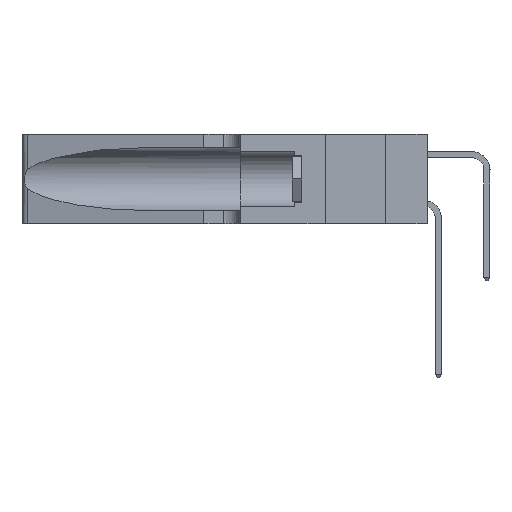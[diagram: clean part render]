
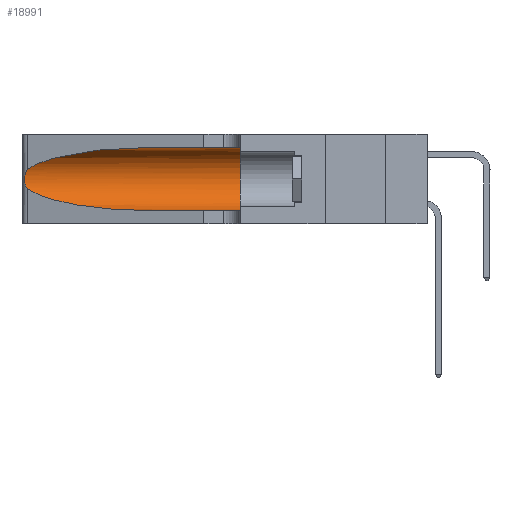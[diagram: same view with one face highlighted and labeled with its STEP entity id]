
A CAD part, left-side view. The second image highlights one B-rep face of the part: STEP entity #18991.
In plain terms, the highlighted cylindrical face has radius 3.308 mm (diameter 6.617 mm), a partial arc.
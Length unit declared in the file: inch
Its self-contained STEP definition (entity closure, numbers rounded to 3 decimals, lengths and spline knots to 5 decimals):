
#11 = EDGE_CURVE ( 'NONE', #18755, #27238, #30736, .T. ) ;
#46 = DIRECTION ( 'NONE',  ( 0., 1., 0. ) ) ;
#856 = CARTESIAN_POINT ( 'NONE',  ( 0.1305, 0.35, 0.05475 ) ) ;
#1956 = CARTESIAN_POINT ( 'NONE',  ( 0.25787, 1.23484, 0.2124 ) ) ;
#2118 = ORIENTED_EDGE ( 'NONE', *, *, #9634, .F. ) ;
#4438 = LINE ( 'NONE', #8211, #25251 ) ;
#4688 = CARTESIAN_POINT ( 'NONE',  ( 0.26018, 1.23835, 0.19895 ) ) ;
#5260 = ORIENTED_EDGE ( 'NONE', *, *, #29958, .T. ) ;
#6292 = CARTESIAN_POINT ( 'NONE',  ( 0.1305, 1.61858, 0.31525 ) ) ;
#6932 = EDGE_CURVE ( 'NONE', #11628, #14616, #9971, .T. ) ;
#7225 = DIRECTION ( 'NONE',  ( 0., 0., -1. ) ) ;
#7465 = CARTESIAN_POINT ( 'NONE',  ( 0.26075, 1.23896, 0.178 ) ) ;
#8211 = CARTESIAN_POINT ( 'NONE',  ( 0.1305, 1.61858, 0.05475 ) ) ;
#8562 = CARTESIAN_POINT ( 'NONE',  ( 0.1305, 0.35, 0.31525 ) ) ;
#8571 = VERTEX_POINT ( 'NONE', #21417 ) ;
#8962 = CARTESIAN_POINT ( 'NONE',  ( 0.1305, 0.35, 0.185 ) ) ;
#9035 = FACE_OUTER_BOUND ( 'NONE', #20756, .T. ) ;
#9094 = CARTESIAN_POINT ( 'NONE',  ( 0.18966, 0.96281, 0.31525 ) ) ;
#9478 = EDGE_CURVE ( 'NONE', #8571, #34686, #26212, .T. ) ;
#9634 = EDGE_CURVE ( 'NONE', #11628, #18755, #11579, .T. ) ;
#9971 =( BOUNDED_CURVE ( )  B_SPLINE_CURVE ( 3, ( #27988, #9094, #11837, #30648 ),
 .UNSPECIFIED., .F., .T. ) 
 B_SPLINE_CURVE_WITH_KNOTS ( ( 4, 4 ),
 ( 1.5708, 2.84003 ),
 .UNSPECIFIED. ) 
 CURVE ( )  GEOMETRIC_REPRESENTATION_ITEM ( )  RATIONAL_B_SPLINE_CURVE ( ( 1., 0.87, 0.87, 1. ) ) 
 REPRESENTATION_ITEM ( '' )  );
#10238 = CARTESIAN_POINT ( 'NONE',  ( 0.25856, 1.23593, 0.16098 ) ) ;
#11579 = LINE ( 'NONE', #6292, #33801 ) ;
#11628 = VERTEX_POINT ( 'NONE', #30861 ) ;
#11837 = CARTESIAN_POINT ( 'NONE',  ( 0.2373, 1.15595, 0.28018 ) ) ;
#12985 = CARTESIAN_POINT ( 'NONE',  ( 0.25639, 1.23186, 0.15144 ) ) ;
#13244 = DIRECTION ( 'NONE',  ( 0., 0., 1. ) ) ;
#13442 = ORIENTED_EDGE ( 'NONE', *, *, #9478, .T. ) ;
#13975 = CARTESIAN_POINT ( 'NONE',  ( 0.18966, 0.96281, 0.05475 ) ) ;
#14616 = VERTEX_POINT ( 'NONE', #15733 ) ;
#14785 = B_SPLINE_CURVE_WITH_KNOTS ( 'NONE', 3,
 ( #23559, #28979, #18248, #1956, #20982, #4688, #23675, #7465, #26421, #10238, #29095, #12985, #31745, #15682 ),
 .UNSPECIFIED., .F., .F.,
 ( 4, 2, 2, 2, 2, 2, 4 ),
 ( 0., 0.00027, 0.00053, 0.00107, 0.0016, 0.00187, 0.00214 ),
 .UNSPECIFIED. ) ;
#14824 = ORIENTED_EDGE ( 'NONE', *, *, #29503, .T. ) ;
#14878 = AXIS2_PLACEMENT_3D ( 'NONE', #8962, #46, #13244 ) ;
#15682 = CARTESIAN_POINT ( 'NONE',  ( 0.25487, 1.22718, 0.14631 ) ) ;
#15733 = CARTESIAN_POINT ( 'NONE',  ( 0.25487, 1.22718, 0.22369 ) ) ;
#16497 = DIRECTION ( 'NONE',  ( 0., -1., 0. ) ) ;
#18018 = CARTESIAN_POINT ( 'NONE',  ( 0.1305, 1.61858, 0.185 ) ) ;
#18248 = CARTESIAN_POINT ( 'NONE',  ( 0.25639, 1.23184, 0.21858 ) ) ;
#18755 = VERTEX_POINT ( 'NONE', #8562 ) ;
#18762 = CARTESIAN_POINT ( 'NONE',  ( 0.1305, 0.72297, 0.05475 ) ) ;
#18910 = AXIS2_PLACEMENT_3D ( 'NONE', #18018, #23454, #7225 ) ;
#18991 = ADVANCED_FACE ( 'NONE', ( #9035 ), #28871, .F. ) ;
#20756 = EDGE_LOOP ( 'NONE', ( #28649, #5260, #13442, #14824, #24135, #2118 ) ) ;
#20982 = CARTESIAN_POINT ( 'NONE',  ( 0.25854, 1.2359, 0.20912 ) ) ;
#21417 = CARTESIAN_POINT ( 'NONE',  ( 0.25487, 1.22718, 0.14631 ) ) ;
#23454 = DIRECTION ( 'NONE',  ( 0., -1., 0. ) ) ;
#23559 = CARTESIAN_POINT ( 'NONE',  ( 0.25487, 1.22718, 0.22369 ) ) ;
#23675 = CARTESIAN_POINT ( 'NONE',  ( 0.26075, 1.23896, 0.19203 ) ) ;
#24135 = ORIENTED_EDGE ( 'NONE', *, *, #11, .F. ) ;
#25251 = VECTOR ( 'NONE', #16497, 39.37008 ) ;
#26212 =( BOUNDED_CURVE ( )  B_SPLINE_CURVE ( 3, ( #27394, #30055, #13975, #32710 ),
 .UNSPECIFIED., .F., .T. ) 
 B_SPLINE_CURVE_WITH_KNOTS ( ( 4, 4 ),
 ( 3.44316, 4.71239 ),
 .UNSPECIFIED. ) 
 CURVE ( )  GEOMETRIC_REPRESENTATION_ITEM ( )  RATIONAL_B_SPLINE_CURVE ( ( 1., 0.87, 0.87, 1. ) ) 
 REPRESENTATION_ITEM ( '' )  );
#26421 = CARTESIAN_POINT ( 'NONE',  ( 0.26017, 1.23833, 0.17102 ) ) ;
#27238 = VERTEX_POINT ( 'NONE', #856 ) ;
#27394 = CARTESIAN_POINT ( 'NONE',  ( 0.25487, 1.22718, 0.14631 ) ) ;
#27988 = CARTESIAN_POINT ( 'NONE',  ( 0.1305, 0.72297, 0.31525 ) ) ;
#28649 = ORIENTED_EDGE ( 'NONE', *, *, #6932, .T. ) ;
#28871 = CYLINDRICAL_SURFACE ( 'NONE', #18910, 0.13025 ) ;
#28979 = CARTESIAN_POINT ( 'NONE',  ( 0.25555, 1.22994, 0.2215 ) ) ;
#29095 = CARTESIAN_POINT ( 'NONE',  ( 0.25789, 1.23486, 0.15765 ) ) ;
#29503 = EDGE_CURVE ( 'NONE', #34686, #27238, #4438, .T. ) ;
#29958 = EDGE_CURVE ( 'NONE', #14616, #8571, #14785, .T. ) ;
#30055 = CARTESIAN_POINT ( 'NONE',  ( 0.2373, 1.15595, 0.08982 ) ) ;
#30637 = DIRECTION ( 'NONE',  ( 0., -1., 0. ) ) ;
#30648 = CARTESIAN_POINT ( 'NONE',  ( 0.25487, 1.22718, 0.22369 ) ) ;
#30736 = CIRCLE ( 'NONE', #14878, 0.13025 ) ;
#30861 = CARTESIAN_POINT ( 'NONE',  ( 0.1305, 0.72297, 0.31525 ) ) ;
#31745 = CARTESIAN_POINT ( 'NONE',  ( 0.25555, 1.22993, 0.14849 ) ) ;
#32710 = CARTESIAN_POINT ( 'NONE',  ( 0.1305, 0.72297, 0.05475 ) ) ;
#33801 = VECTOR ( 'NONE', #30637, 39.37008 ) ;
#34686 = VERTEX_POINT ( 'NONE', #18762 ) ;
